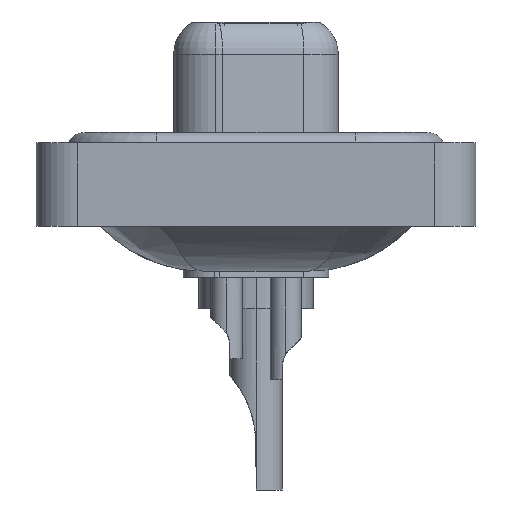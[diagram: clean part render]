
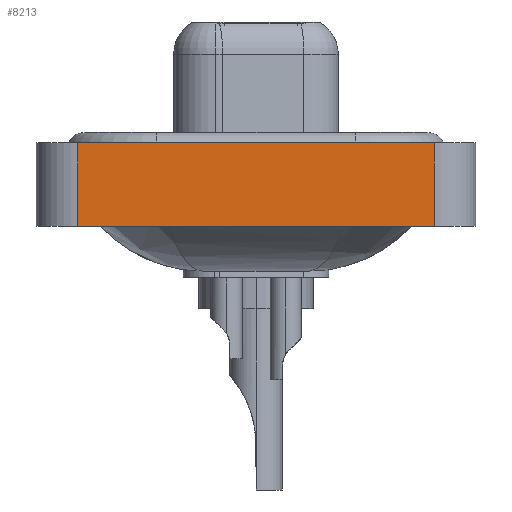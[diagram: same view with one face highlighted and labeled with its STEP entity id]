
A CAD part, left-side view. The second image highlights one B-rep face of the part: STEP entity #8213.
In plain terms, the highlighted planar face has unit normal (-1, 0, 0).
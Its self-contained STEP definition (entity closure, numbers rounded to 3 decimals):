
#836 = VERTEX_POINT ( 'NONE', #8995 ) ;
#1359 = VECTOR ( 'NONE', #10987, 1000. ) ;
#1504 = FACE_OUTER_BOUND ( 'NONE', #4714, .T. ) ;
#1736 = ORIENTED_EDGE ( 'NONE', *, *, #5617, .T. ) ;
#2613 = DIRECTION ( 'NONE',  ( -1., 0., 0. ) ) ;
#3665 = ORIENTED_EDGE ( 'NONE', *, *, #18619, .T. ) ;
#4606 = LINE ( 'NONE', #18717, #1359 ) ;
#4614 = VERTEX_POINT ( 'NONE', #18503 ) ;
#4690 = ORIENTED_EDGE ( 'NONE', *, *, #16779, .F. ) ;
#4714 = EDGE_LOOP ( 'NONE', ( #3665, #4690, #8599, #1736 ) ) ;
#5617 = EDGE_CURVE ( 'NONE', #836, #7106, #8780, .T. ) ;
#5900 = CARTESIAN_POINT ( 'NONE',  ( -7.25, -8.55, 0.4 ) ) ;
#6223 = LINE ( 'NONE', #9360, #16347 ) ;
#7106 = VERTEX_POINT ( 'NONE', #9786 ) ;
#7635 = CARTESIAN_POINT ( 'NONE',  ( -7.25, -8.55, -3.6 ) ) ;
#8213 = ADVANCED_FACE ( 'NONE', ( #1504 ), #10485, .T. ) ;
#8599 = ORIENTED_EDGE ( 'NONE', *, *, #16415, .F. ) ;
#8780 = LINE ( 'NONE', #8878, #14201 ) ;
#8878 = CARTESIAN_POINT ( 'NONE',  ( -7.25, -8.55, -3.6 ) ) ;
#8995 = CARTESIAN_POINT ( 'NONE',  ( -7.25, 8.55, -3.6 ) ) ;
#9360 = CARTESIAN_POINT ( 'NONE',  ( -7.25, -8.55, -3.6 ) ) ;
#9786 = CARTESIAN_POINT ( 'NONE',  ( -7.25, -8.55, -3.6 ) ) ;
#10485 = PLANE ( 'NONE',  #16590 ) ;
#10987 = DIRECTION ( 'NONE',  ( 0., 0., 1. ) ) ;
#12077 = DIRECTION ( 'NONE',  ( 0., -1., 0. ) ) ;
#12084 = VERTEX_POINT ( 'NONE', #18373 ) ;
#13428 = DIRECTION ( 'NONE',  ( 0., 0., 1. ) ) ;
#13458 = DIRECTION ( 'NONE',  ( 0., -1., 0. ) ) ;
#14201 = VECTOR ( 'NONE', #13458, 1000. ) ;
#14500 = DIRECTION ( 'NONE',  ( 0., 0., 1. ) ) ;
#16347 = VECTOR ( 'NONE', #14500, 1000. ) ;
#16415 = EDGE_CURVE ( 'NONE', #836, #12084, #4606, .T. ) ;
#16590 = AXIS2_PLACEMENT_3D ( 'NONE', #7635, #2613, #13428 ) ;
#16779 = EDGE_CURVE ( 'NONE', #12084, #4614, #19718, .T. ) ;
#17117 = VECTOR ( 'NONE', #12077, 1000. ) ;
#18373 = CARTESIAN_POINT ( 'NONE',  ( -7.25, 8.55, 0.4 ) ) ;
#18503 = CARTESIAN_POINT ( 'NONE',  ( -7.25, -8.55, 0.4 ) ) ;
#18619 = EDGE_CURVE ( 'NONE', #7106, #4614, #6223, .T. ) ;
#18717 = CARTESIAN_POINT ( 'NONE',  ( -7.25, 8.55, -3.6 ) ) ;
#19718 = LINE ( 'NONE', #5900, #17117 ) ;
